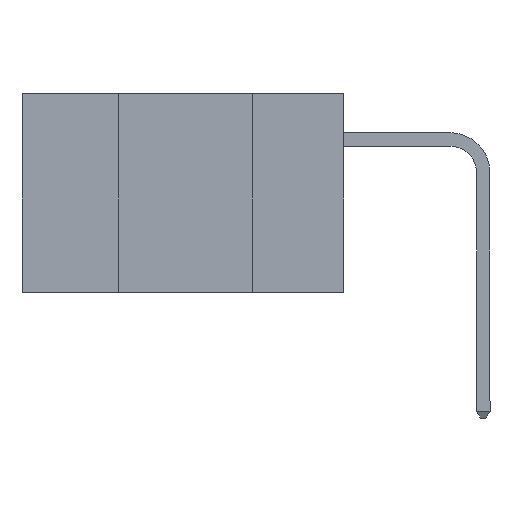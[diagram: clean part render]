
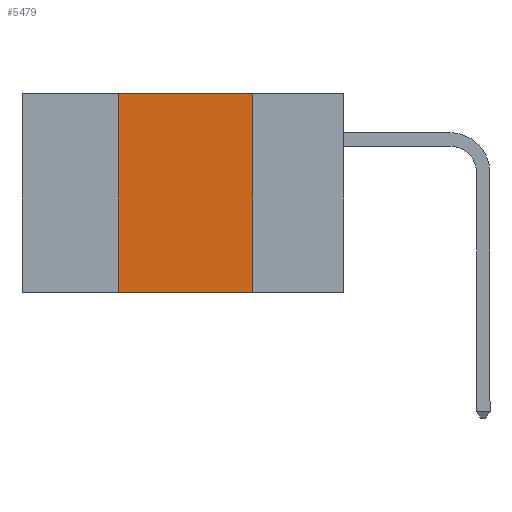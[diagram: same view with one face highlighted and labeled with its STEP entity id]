
A CAD part, left-side view. The second image highlights one B-rep face of the part: STEP entity #5479.
In plain terms, the highlighted planar face has unit normal (-1, 0, 0).
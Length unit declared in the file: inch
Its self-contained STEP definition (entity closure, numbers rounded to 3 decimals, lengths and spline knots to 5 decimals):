
#104 = LINE ( 'NONE', #6158, #7110 ) ;
#126 = CARTESIAN_POINT ( 'NONE',  ( 0., 0.17, -0.37 ) ) ;
#263 = DIRECTION ( 'NONE',  ( 0., 0., -1. ) ) ;
#316 = EDGE_CURVE ( 'NONE', #4388, #5481, #8123, .T. ) ;
#343 = AXIS2_PLACEMENT_3D ( 'NONE', #3393, #5438, #263 ) ;
#359 = CARTESIAN_POINT ( 'NONE',  ( 0., 0.42, -0.37 ) ) ;
#887 = VECTOR ( 'NONE', #1272, 39.37008 ) ;
#1272 = DIRECTION ( 'NONE',  ( 0., -1., 0. ) ) ;
#1290 = EDGE_CURVE ( 'NONE', #7950, #5481, #104, .T. ) ;
#1364 = DIRECTION ( 'NONE',  ( 0., 0., 1. ) ) ;
#1437 = EDGE_CURVE ( 'NONE', #7204, #7950, #2779, .T. ) ;
#1563 = ORIENTED_EDGE ( 'NONE', *, *, #1290, .F. ) ;
#1914 = EDGE_LOOP ( 'NONE', ( #1563, #3541, #2583, #5860 ) ) ;
#2430 = VECTOR ( 'NONE', #1364, 39.37008 ) ;
#2438 = CARTESIAN_POINT ( 'NONE',  ( 0., 0.42, 0. ) ) ;
#2446 = PLANE ( 'NONE',  #343 ) ;
#2548 = EDGE_CURVE ( 'NONE', #4388, #7204, #6403, .T. ) ;
#2583 = ORIENTED_EDGE ( 'NONE', *, *, #2548, .F. ) ;
#2779 = LINE ( 'NONE', #5760, #887 ) ;
#2997 = VECTOR ( 'NONE', #8428, 39.37008 ) ;
#3393 = CARTESIAN_POINT ( 'NONE',  ( 0., 0.6, 0. ) ) ;
#3541 = ORIENTED_EDGE ( 'NONE', *, *, #1437, .F. ) ;
#3948 = CARTESIAN_POINT ( 'NONE',  ( 0., 0.6, -0.37 ) ) ;
#3998 = CARTESIAN_POINT ( 'NONE',  ( 0., 0.17, 0. ) ) ;
#4388 = VERTEX_POINT ( 'NONE', #6369 ) ;
#5438 = DIRECTION ( 'NONE',  ( 1., 0., 0. ) ) ;
#5479 = ADVANCED_FACE ( 'NONE', ( #6754 ), #2446, .F. ) ;
#5481 = VERTEX_POINT ( 'NONE', #126 ) ;
#5729 = DIRECTION ( 'NONE',  ( 0., 0., -1. ) ) ;
#5760 = CARTESIAN_POINT ( 'NONE',  ( 0., 0.6, 0. ) ) ;
#5860 = ORIENTED_EDGE ( 'NONE', *, *, #316, .T. ) ;
#6158 = CARTESIAN_POINT ( 'NONE',  ( 0., 0.17, -0.37 ) ) ;
#6369 = CARTESIAN_POINT ( 'NONE',  ( 0., 0.42, -0.37 ) ) ;
#6403 = LINE ( 'NONE', #359, #2430 ) ;
#6754 = FACE_OUTER_BOUND ( 'NONE', #1914, .T. ) ;
#7110 = VECTOR ( 'NONE', #5729, 39.37008 ) ;
#7204 = VERTEX_POINT ( 'NONE', #2438 ) ;
#7950 = VERTEX_POINT ( 'NONE', #3998 ) ;
#8123 = LINE ( 'NONE', #3948, #2997 ) ;
#8428 = DIRECTION ( 'NONE',  ( 0., -1., 0. ) ) ;
